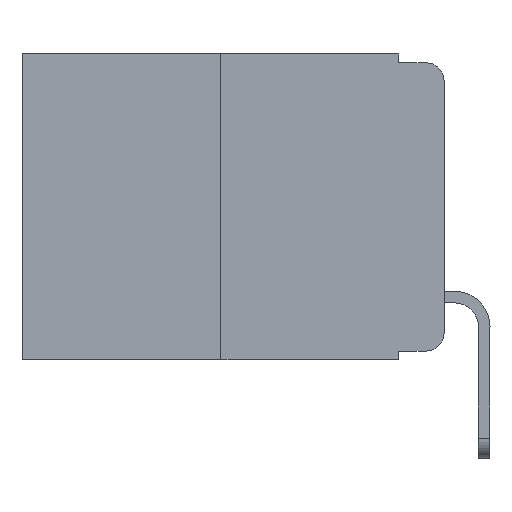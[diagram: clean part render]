
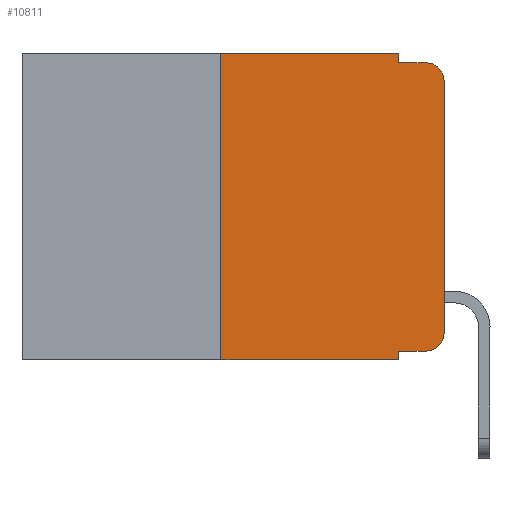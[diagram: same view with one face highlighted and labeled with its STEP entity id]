
A CAD part, left-side view. The second image highlights one B-rep face of the part: STEP entity #10811.
In plain terms, the highlighted planar face has unit normal (-1, 0, 0).
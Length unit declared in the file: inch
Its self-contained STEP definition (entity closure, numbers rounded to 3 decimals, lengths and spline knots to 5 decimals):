
#34 = LINE ( 'NONE', #8737, #12682 ) ;
#144 = CARTESIAN_POINT ( 'NONE',  ( 0., 0., 0. ) ) ;
#193 = DIRECTION ( 'NONE',  ( 0., 0., 1. ) ) ;
#455 = EDGE_CURVE ( 'NONE', #11449, #9011, #916, .T. ) ;
#491 = DIRECTION ( 'NONE',  ( 0., 0., -1. ) ) ;
#551 = DIRECTION ( 'NONE',  ( 0., 0., -1. ) ) ;
#574 = CARTESIAN_POINT ( 'NONE',  ( 0., 0.02, -0.01 ) ) ;
#645 = VERTEX_POINT ( 'NONE', #1274 ) ;
#837 = AXIS2_PLACEMENT_3D ( 'NONE', #12154, #12194, #8170 ) ;
#878 = VECTOR ( 'NONE', #5886, 39.37008 ) ;
#916 = LINE ( 'NONE', #7857, #2961 ) ;
#1106 = CIRCLE ( 'NONE', #13068, 0.02 ) ;
#1274 = CARTESIAN_POINT ( 'NONE',  ( 0., 0.25, 0. ) ) ;
#1307 = EDGE_CURVE ( 'NONE', #9011, #7487, #7547, .T. ) ;
#1350 = DIRECTION ( 'NONE',  ( 0., -1., 0. ) ) ;
#1580 = ORIENTED_EDGE ( 'NONE', *, *, #9495, .T. ) ;
#1699 = FACE_OUTER_BOUND ( 'NONE', #8125, .T. ) ;
#1824 = VERTEX_POINT ( 'NONE', #3612 ) ;
#2157 = EDGE_CURVE ( 'NONE', #7326, #1824, #5783, .T. ) ;
#2176 = DIRECTION ( 'NONE',  ( 0., 0., 1. ) ) ;
#2606 = CARTESIAN_POINT ( 'NONE',  ( 0., 0.051, -0.01 ) ) ;
#2644 = CARTESIAN_POINT ( 'NONE',  ( 0., 0., -0.313 ) ) ;
#2677 = CARTESIAN_POINT ( 'NONE',  ( 0., 0.02, -0.03 ) ) ;
#2925 = ORIENTED_EDGE ( 'NONE', *, *, #1307, .T. ) ;
#2956 = VERTEX_POINT ( 'NONE', #12583 ) ;
#2961 = VECTOR ( 'NONE', #6783, 39.37008 ) ;
#3331 = DIRECTION ( 'NONE',  ( 1., 0., 0. ) ) ;
#3386 = VECTOR ( 'NONE', #2176, 39.37008 ) ;
#3612 = CARTESIAN_POINT ( 'NONE',  ( 0., 0.051, -0.343 ) ) ;
#3677 = CARTESIAN_POINT ( 'NONE',  ( 0., 0.473, 0. ) ) ;
#3693 = EDGE_CURVE ( 'NONE', #5599, #7393, #6070, .T. ) ;
#4026 = ORIENTED_EDGE ( 'NONE', *, *, #4616, .F. ) ;
#4254 = CARTESIAN_POINT ( 'NONE',  ( 0., 0.051, -0.333 ) ) ;
#4287 = EDGE_CURVE ( 'NONE', #7487, #4516, #4967, .T. ) ;
#4352 = PLANE ( 'NONE',  #6553 ) ;
#4516 = VERTEX_POINT ( 'NONE', #9349 ) ;
#4545 = ORIENTED_EDGE ( 'NONE', *, *, #3693, .F. ) ;
#4616 = EDGE_CURVE ( 'NONE', #2956, #5599, #13028, .T. ) ;
#4628 = EDGE_CURVE ( 'NONE', #645, #2956, #6217, .T. ) ;
#4912 = CARTESIAN_POINT ( 'NONE',  ( 0., 0.051, -0.01 ) ) ;
#4967 = LINE ( 'NONE', #144, #3386 ) ;
#5251 = ORIENTED_EDGE ( 'NONE', *, *, #4628, .F. ) ;
#5277 = ORIENTED_EDGE ( 'NONE', *, *, #455, .T. ) ;
#5329 = CARTESIAN_POINT ( 'NONE',  ( 0., 0.25, -0.343 ) ) ;
#5599 = VERTEX_POINT ( 'NONE', #2606 ) ;
#5783 = LINE ( 'NONE', #6363, #11968 ) ;
#5886 = DIRECTION ( 'NONE',  ( 0., -1., 0. ) ) ;
#5983 = VECTOR ( 'NONE', #193, 39.37008 ) ;
#6070 = LINE ( 'NONE', #4912, #878 ) ;
#6106 = ORIENTED_EDGE ( 'NONE', *, *, #12820, .F. ) ;
#6217 = LINE ( 'NONE', #3677, #10018 ) ;
#6363 = CARTESIAN_POINT ( 'NONE',  ( 0., 0.473, -0.343 ) ) ;
#6553 = AXIS2_PLACEMENT_3D ( 'NONE', #10264, #3331, #8257 ) ;
#6783 = DIRECTION ( 'NONE',  ( 0., -1., 0. ) ) ;
#7032 = CARTESIAN_POINT ( 'NONE',  ( 0., 0.02, -0.333 ) ) ;
#7326 = VERTEX_POINT ( 'NONE', #5329 ) ;
#7393 = VERTEX_POINT ( 'NONE', #574 ) ;
#7444 = ORIENTED_EDGE ( 'NONE', *, *, #10805, .F. ) ;
#7487 = VERTEX_POINT ( 'NONE', #2644 ) ;
#7547 = CIRCLE ( 'NONE', #837, 0.02 ) ;
#7744 = DIRECTION ( 'NONE',  ( 0., 0., -1. ) ) ;
#7857 = CARTESIAN_POINT ( 'NONE',  ( 0., 0.051, -0.333 ) ) ;
#8024 = LINE ( 'NONE', #9234, #5983 ) ;
#8077 = ORIENTED_EDGE ( 'NONE', *, *, #4287, .T. ) ;
#8125 = EDGE_LOOP ( 'NONE', ( #8077, #1580, #4545, #4026, #5251, #7444, #12793, #6106, #5277, #2925 ) ) ;
#8170 = DIRECTION ( 'NONE',  ( 0., 0., -1. ) ) ;
#8257 = DIRECTION ( 'NONE',  ( 0., 0., -1. ) ) ;
#8737 = CARTESIAN_POINT ( 'NONE',  ( 0., 0.051, 0. ) ) ;
#9011 = VERTEX_POINT ( 'NONE', #7032 ) ;
#9234 = CARTESIAN_POINT ( 'NONE',  ( 0., 0.25, 0. ) ) ;
#9349 = CARTESIAN_POINT ( 'NONE',  ( 0., 0., -0.03 ) ) ;
#9495 = EDGE_CURVE ( 'NONE', #4516, #7393, #1106, .T. ) ;
#9738 = DIRECTION ( 'NONE',  ( -1., 0., 0. ) ) ;
#10018 = VECTOR ( 'NONE', #11622, 39.37008 ) ;
#10264 = CARTESIAN_POINT ( 'NONE',  ( 0., 0.473, 0. ) ) ;
#10695 = CARTESIAN_POINT ( 'NONE',  ( 0., 0.051, 0. ) ) ;
#10805 = EDGE_CURVE ( 'NONE', #7326, #645, #8024, .T. ) ;
#10811 = ADVANCED_FACE ( 'NONE', ( #1699 ), #4352, .F. ) ;
#11449 = VERTEX_POINT ( 'NONE', #4254 ) ;
#11612 = VECTOR ( 'NONE', #491, 39.37008 ) ;
#11622 = DIRECTION ( 'NONE',  ( 0., -1., 0. ) ) ;
#11968 = VECTOR ( 'NONE', #1350, 39.37008 ) ;
#12154 = CARTESIAN_POINT ( 'NONE',  ( 0., 0.02, -0.313 ) ) ;
#12194 = DIRECTION ( 'NONE',  ( -1., 0., 0. ) ) ;
#12583 = CARTESIAN_POINT ( 'NONE',  ( 0., 0.051, 0. ) ) ;
#12682 = VECTOR ( 'NONE', #551, 39.37008 ) ;
#12793 = ORIENTED_EDGE ( 'NONE', *, *, #2157, .T. ) ;
#12820 = EDGE_CURVE ( 'NONE', #11449, #1824, #34, .T. ) ;
#13028 = LINE ( 'NONE', #10695, #11612 ) ;
#13068 = AXIS2_PLACEMENT_3D ( 'NONE', #2677, #9738, #7744 ) ;
